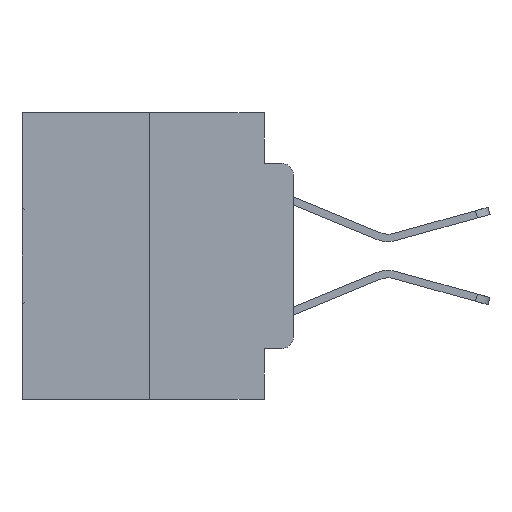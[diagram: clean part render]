
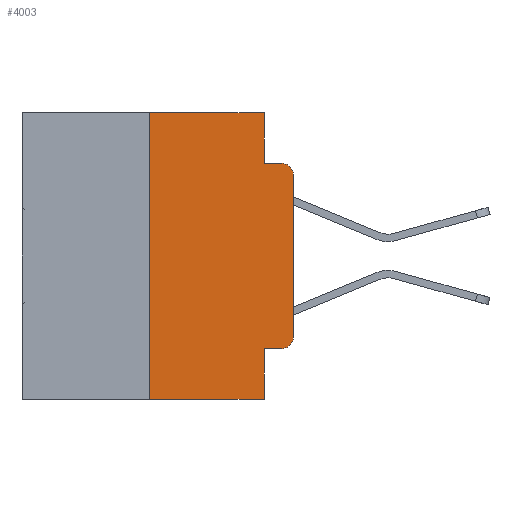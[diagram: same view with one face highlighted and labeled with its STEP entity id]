
A CAD part, left-side view. The second image highlights one B-rep face of the part: STEP entity #4003.
In plain terms, the highlighted planar face has unit normal (-1, 0, 0).
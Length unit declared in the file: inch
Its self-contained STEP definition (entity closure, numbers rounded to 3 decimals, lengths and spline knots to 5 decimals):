
#467 = LINE ( 'NONE', #16175, #6001 ) ;
#1012 = CARTESIAN_POINT ( 'NONE',  ( 0., 0.02, -0.3915 ) ) ;
#1385 = CARTESIAN_POINT ( 'NONE',  ( 0., 0., -0.3915 ) ) ;
#1586 = CIRCLE ( 'NONE', #16562, 0.02 ) ;
#1763 = EDGE_CURVE ( 'NONE', #2807, #22616, #8550, .T. ) ;
#1812 = FACE_OUTER_BOUND ( 'NONE', #20717, .T. ) ;
#1848 = DIRECTION ( 'NONE',  ( 0., 0., 1. ) ) ;
#1930 = CARTESIAN_POINT ( 'NONE',  ( 0., 0.051, -0.5 ) ) ;
#1981 = CARTESIAN_POINT ( 'NONE',  ( 0., 0.051, -0.4115 ) ) ;
#2455 = DIRECTION ( 'NONE',  ( 0., 0., 1. ) ) ;
#2557 = CARTESIAN_POINT ( 'NONE',  ( 0., 0.25, 0. ) ) ;
#2807 = VERTEX_POINT ( 'NONE', #5911 ) ;
#2829 = ORIENTED_EDGE ( 'NONE', *, *, #17376, .F. ) ;
#3359 = DIRECTION ( 'NONE',  ( 0., 0., -1. ) ) ;
#4003 = ADVANCED_FACE ( 'NONE', ( #1812 ), #8974, .F. ) ;
#4417 = CARTESIAN_POINT ( 'NONE',  ( 0., 0.02, -0.1085 ) ) ;
#4506 = DIRECTION ( 'NONE',  ( 1., 0., 0. ) ) ;
#4578 = LINE ( 'NONE', #2557, #23451 ) ;
#4890 = CARTESIAN_POINT ( 'NONE',  ( 0., 0.051, 0. ) ) ;
#5911 = CARTESIAN_POINT ( 'NONE',  ( 0., 0.25, 0. ) ) ;
#6001 = VECTOR ( 'NONE', #18554, 39.37008 ) ;
#6345 = CARTESIAN_POINT ( 'NONE',  ( 0., 0.051, -0.0885 ) ) ;
#6592 = DIRECTION ( 'NONE',  ( 0., -1., 0. ) ) ;
#6680 = AXIS2_PLACEMENT_3D ( 'NONE', #28553, #4506, #23940 ) ;
#6764 = DIRECTION ( 'NONE',  ( 0., 0., -1. ) ) ;
#6856 = VERTEX_POINT ( 'NONE', #1930 ) ;
#6991 = VERTEX_POINT ( 'NONE', #23669 ) ;
#7273 = ORIENTED_EDGE ( 'NONE', *, *, #23757, .T. ) ;
#8434 = ORIENTED_EDGE ( 'NONE', *, *, #15778, .F. ) ;
#8550 = LINE ( 'NONE', #25892, #20409 ) ;
#8654 = CARTESIAN_POINT ( 'NONE',  ( 0., 0.25, -0.5 ) ) ;
#8712 = DIRECTION ( 'NONE',  ( 0., -1., 0. ) ) ;
#8974 = PLANE ( 'NONE',  #6680 ) ;
#9756 = LINE ( 'NONE', #30098, #27896 ) ;
#10998 = ORIENTED_EDGE ( 'NONE', *, *, #17784, .T. ) ;
#11020 = EDGE_CURVE ( 'NONE', #23865, #20739, #29144, .T. ) ;
#11616 = VECTOR ( 'NONE', #26619, 39.37008 ) ;
#12083 = ORIENTED_EDGE ( 'NONE', *, *, #22151, .F. ) ;
#12611 = EDGE_CURVE ( 'NONE', #27944, #23865, #18865, .T. ) ;
#14714 = ORIENTED_EDGE ( 'NONE', *, *, #12611, .T. ) ;
#14813 = CARTESIAN_POINT ( 'NONE',  ( 0., 0.051, 0. ) ) ;
#15041 = ORIENTED_EDGE ( 'NONE', *, *, #26880, .T. ) ;
#15778 = EDGE_CURVE ( 'NONE', #27944, #6856, #30420, .T. ) ;
#16175 = CARTESIAN_POINT ( 'NONE',  ( 0., 0.473, -0.5 ) ) ;
#16562 = AXIS2_PLACEMENT_3D ( 'NONE', #4417, #20953, #6764 ) ;
#17118 = VERTEX_POINT ( 'NONE', #8654 ) ;
#17376 = EDGE_CURVE ( 'NONE', #17118, #2807, #4578, .T. ) ;
#17532 = DIRECTION ( 'NONE',  ( -1., 0., 0. ) ) ;
#17541 = VERTEX_POINT ( 'NONE', #22427 ) ;
#17784 = EDGE_CURVE ( 'NONE', #17118, #6856, #467, .T. ) ;
#18279 = DIRECTION ( 'NONE',  ( 0., 0., -1. ) ) ;
#18478 = CARTESIAN_POINT ( 'NONE',  ( 0., 0.051, -0.4115 ) ) ;
#18554 = DIRECTION ( 'NONE',  ( 0., -1., 0. ) ) ;
#18865 = LINE ( 'NONE', #18478, #24441 ) ;
#18949 = EDGE_CURVE ( 'NONE', #22616, #17541, #26257, .T. ) ;
#19969 = VECTOR ( 'NONE', #18279, 39.37008 ) ;
#20409 = VECTOR ( 'NONE', #23948, 39.37008 ) ;
#20717 = EDGE_LOOP ( 'NONE', ( #15041, #7273, #12083, #29415, #23221, #2829, #10998, #8434, #14714, #28028 ) ) ;
#20739 = VERTEX_POINT ( 'NONE', #1385 ) ;
#20953 = DIRECTION ( 'NONE',  ( -1., 0., 0. ) ) ;
#21112 = AXIS2_PLACEMENT_3D ( 'NONE', #1012, #17532, #3359 ) ;
#22151 = EDGE_CURVE ( 'NONE', #17541, #6991, #27505, .T. ) ;
#22427 = CARTESIAN_POINT ( 'NONE',  ( 0., 0.051, -0.0885 ) ) ;
#22616 = VERTEX_POINT ( 'NONE', #4890 ) ;
#23221 = ORIENTED_EDGE ( 'NONE', *, *, #1763, .F. ) ;
#23451 = VECTOR ( 'NONE', #2455, 39.37008 ) ;
#23669 = CARTESIAN_POINT ( 'NONE',  ( 0., 0.02, -0.0885 ) ) ;
#23757 = EDGE_CURVE ( 'NONE', #25573, #6991, #1586, .T. ) ;
#23865 = VERTEX_POINT ( 'NONE', #30570 ) ;
#23940 = DIRECTION ( 'NONE',  ( 0., 0., -1. ) ) ;
#23948 = DIRECTION ( 'NONE',  ( 0., -1., 0. ) ) ;
#24441 = VECTOR ( 'NONE', #6592, 39.37008 ) ;
#24878 = CARTESIAN_POINT ( 'NONE',  ( 0., 0., -0.1085 ) ) ;
#25238 = CARTESIAN_POINT ( 'NONE',  ( 0., 0.051, 0. ) ) ;
#25573 = VERTEX_POINT ( 'NONE', #24878 ) ;
#25892 = CARTESIAN_POINT ( 'NONE',  ( 0., 0.473, 0. ) ) ;
#26257 = LINE ( 'NONE', #25238, #19969 ) ;
#26619 = DIRECTION ( 'NONE',  ( 0., 0., -1. ) ) ;
#26779 = VECTOR ( 'NONE', #8712, 39.37008 ) ;
#26880 = EDGE_CURVE ( 'NONE', #20739, #25573, #9756, .T. ) ;
#27505 = LINE ( 'NONE', #6345, #26779 ) ;
#27896 = VECTOR ( 'NONE', #1848, 39.37008 ) ;
#27944 = VERTEX_POINT ( 'NONE', #1981 ) ;
#28028 = ORIENTED_EDGE ( 'NONE', *, *, #11020, .T. ) ;
#28553 = CARTESIAN_POINT ( 'NONE',  ( 0., 0.473, 0. ) ) ;
#29144 = CIRCLE ( 'NONE', #21112, 0.02 ) ;
#29415 = ORIENTED_EDGE ( 'NONE', *, *, #18949, .F. ) ;
#30098 = CARTESIAN_POINT ( 'NONE',  ( 0., 0., 0. ) ) ;
#30420 = LINE ( 'NONE', #14813, #11616 ) ;
#30570 = CARTESIAN_POINT ( 'NONE',  ( 0., 0.02, -0.4115 ) ) ;
